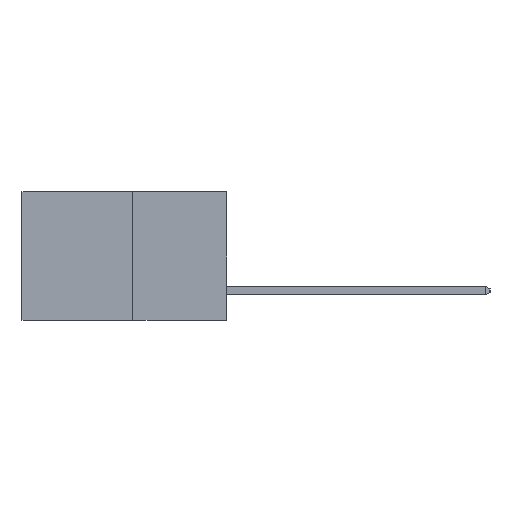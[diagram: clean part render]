
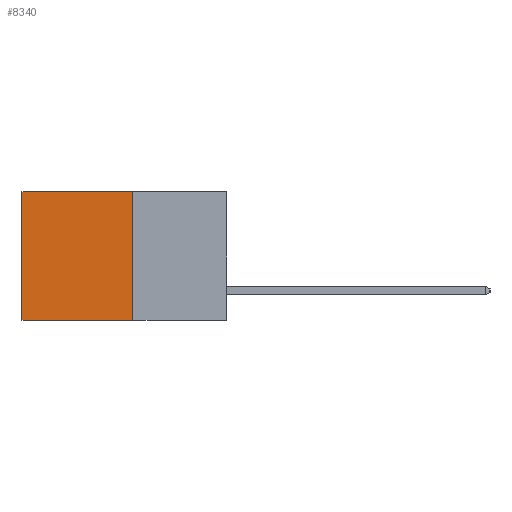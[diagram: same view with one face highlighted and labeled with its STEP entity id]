
A CAD part, left-side view. The second image highlights one B-rep face of the part: STEP entity #8340.
In plain terms, the highlighted planar face has unit normal (-1, 0, 0).
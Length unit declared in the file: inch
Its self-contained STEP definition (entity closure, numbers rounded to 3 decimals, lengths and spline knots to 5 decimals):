
#85 = VERTEX_POINT ( 'NONE', #11906 ) ;
#538 = LINE ( 'NONE', #10616, #8273 ) ;
#951 = VECTOR ( 'NONE', #1252, 39.37008 ) ;
#1081 = DIRECTION ( 'NONE',  ( 0., 1., 0. ) ) ;
#1228 = CARTESIAN_POINT ( 'NONE',  ( 0.277, 0.27, -0.37 ) ) ;
#1252 = DIRECTION ( 'NONE',  ( 0., 1., 0. ) ) ;
#1274 = VECTOR ( 'NONE', #1081, 39.37008 ) ;
#1384 = CARTESIAN_POINT ( 'NONE',  ( 0.277, 0.27, 0. ) ) ;
#2380 = DIRECTION ( 'NONE',  ( 1., 0., 0. ) ) ;
#2854 = LINE ( 'NONE', #7819, #7871 ) ;
#2971 = AXIS2_PLACEMENT_3D ( 'NONE', #9309, #2380, #9348 ) ;
#3076 = VERTEX_POINT ( 'NONE', #1384 ) ;
#3168 = EDGE_LOOP ( 'NONE', ( #4288, #4235, #3523, #3767 ) ) ;
#3523 = ORIENTED_EDGE ( 'NONE', *, *, #5934, .F. ) ;
#3767 = ORIENTED_EDGE ( 'NONE', *, *, #7385, .T. ) ;
#4081 = LINE ( 'NONE', #1228, #1274 ) ;
#4235 = ORIENTED_EDGE ( 'NONE', *, *, #7175, .F. ) ;
#4288 = ORIENTED_EDGE ( 'NONE', *, *, #8086, .T. ) ;
#5062 = CARTESIAN_POINT ( 'NONE',  ( 0.277, 0.59, -0.37 ) ) ;
#5934 = EDGE_CURVE ( 'NONE', #3076, #7435, #538, .T. ) ;
#6361 = LINE ( 'NONE', #7318, #951 ) ;
#7175 = EDGE_CURVE ( 'NONE', #7435, #10842, #4081, .T. ) ;
#7318 = CARTESIAN_POINT ( 'NONE',  ( 0.277, 0.27, 0. ) ) ;
#7385 = EDGE_CURVE ( 'NONE', #3076, #85, #6361, .T. ) ;
#7425 = PLANE ( 'NONE',  #2971 ) ;
#7435 = VERTEX_POINT ( 'NONE', #9340 ) ;
#7550 = FACE_OUTER_BOUND ( 'NONE', #3168, .T. ) ;
#7819 = CARTESIAN_POINT ( 'NONE',  ( 0.277, 0.59, -0.37 ) ) ;
#7871 = VECTOR ( 'NONE', #10565, 39.37008 ) ;
#8086 = EDGE_CURVE ( 'NONE', #85, #10842, #2854, .T. ) ;
#8273 = VECTOR ( 'NONE', #10591, 39.37008 ) ;
#8340 = ADVANCED_FACE ( 'NONE', ( #7550 ), #7425, .F. ) ;
#9309 = CARTESIAN_POINT ( 'NONE',  ( 0.277, 0.27, -0.37 ) ) ;
#9340 = CARTESIAN_POINT ( 'NONE',  ( 0.277, 0.27, -0.37 ) ) ;
#9348 = DIRECTION ( 'NONE',  ( 0., 0., -1. ) ) ;
#10565 = DIRECTION ( 'NONE',  ( 0., 0., -1. ) ) ;
#10591 = DIRECTION ( 'NONE',  ( 0., 0., -1. ) ) ;
#10616 = CARTESIAN_POINT ( 'NONE',  ( 0.277, 0.27, -0.37 ) ) ;
#10842 = VERTEX_POINT ( 'NONE', #5062 ) ;
#11906 = CARTESIAN_POINT ( 'NONE',  ( 0.277, 0.59, 0. ) ) ;
